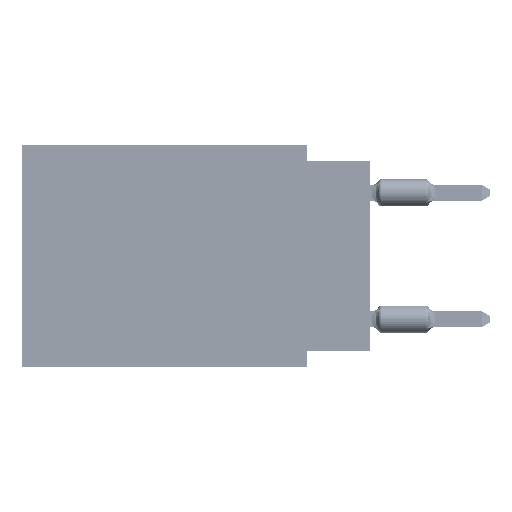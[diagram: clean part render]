
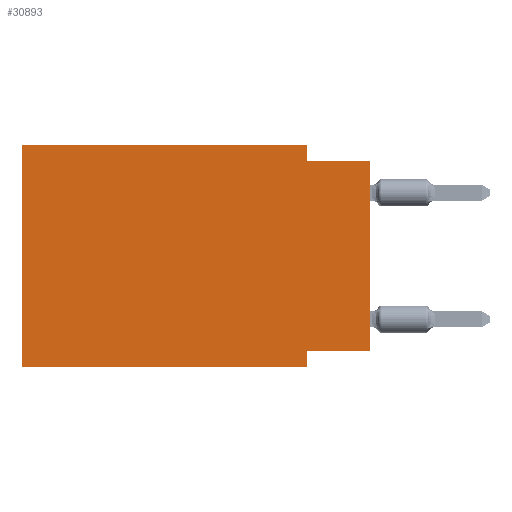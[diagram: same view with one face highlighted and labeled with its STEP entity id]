
A CAD part, left-side view. The second image highlights one B-rep face of the part: STEP entity #30893.
In plain terms, the highlighted planar face has unit normal (-1, 0, 0).
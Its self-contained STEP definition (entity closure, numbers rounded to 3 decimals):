
#2110 = CARTESIAN_POINT ( 'NONE',  ( 0., 2.54, -0.635 ) ) ;
#4095 = FACE_OUTER_BOUND ( 'NONE', #34956, .T. ) ;
#6099 = CARTESIAN_POINT ( 'NONE',  ( 0., 13.97, -8.89 ) ) ;
#6158 = CARTESIAN_POINT ( 'NONE',  ( 0., 2.54, 0. ) ) ;
#8607 = ORIENTED_EDGE ( 'NONE', *, *, #38742, .F. ) ;
#10817 = DIRECTION ( 'NONE',  ( 0., 0., -1. ) ) ;
#11396 = ORIENTED_EDGE ( 'NONE', *, *, #22420, .F. ) ;
#11753 = VECTOR ( 'NONE', #76436, 1000. ) ;
#12041 = LINE ( 'NONE', #6158, #82120 ) ;
#13299 = CARTESIAN_POINT ( 'NONE',  ( 0., 0., -0.635 ) ) ;
#13456 = DIRECTION ( 'NONE',  ( 0., -1., 0. ) ) ;
#13881 = LINE ( 'NONE', #44991, #46534 ) ;
#14516 = VERTEX_POINT ( 'NONE', #49540 ) ;
#15946 = VECTOR ( 'NONE', #69923, 1000. ) ;
#16169 = CARTESIAN_POINT ( 'NONE',  ( 0., 2.54, 0. ) ) ;
#17230 = LINE ( 'NONE', #75221, #55458 ) ;
#17736 = LINE ( 'NONE', #56386, #31628 ) ;
#20654 = CARTESIAN_POINT ( 'NONE',  ( 0., 2.54, -8.89 ) ) ;
#22420 = EDGE_CURVE ( 'NONE', #79474, #53829, #17230, .T. ) ;
#25163 = CARTESIAN_POINT ( 'NONE',  ( 0., 13.97, -8.89 ) ) ;
#25409 = VECTOR ( 'NONE', #31245, 1000. ) ;
#25682 = CARTESIAN_POINT ( 'NONE',  ( 0., 13.97, 0. ) ) ;
#26259 = EDGE_CURVE ( 'NONE', #60961, #70856, #13881, .T. ) ;
#28973 = EDGE_CURVE ( 'NONE', #14516, #79474, #46061, .T. ) ;
#29222 = ORIENTED_EDGE ( 'NONE', *, *, #26259, .F. ) ;
#29746 = PLANE ( 'NONE',  #76397 ) ;
#29866 = DIRECTION ( 'NONE',  ( 0., 0., -1. ) ) ;
#30893 = ADVANCED_FACE ( 'NONE', ( #4095 ), #29746, .F. ) ;
#30972 = DIRECTION ( 'NONE',  ( 0., 0., -1. ) ) ;
#31245 = DIRECTION ( 'NONE',  ( 0., -1., 0. ) ) ;
#31508 = ORIENTED_EDGE ( 'NONE', *, *, #77738, .T. ) ;
#31628 = VECTOR ( 'NONE', #68995, 1000. ) ;
#34956 = EDGE_LOOP ( 'NONE', ( #69501, #36332, #8607, #29222, #40381, #31508, #11396, #66861 ) ) ;
#36332 = ORIENTED_EDGE ( 'NONE', *, *, #47498, .F. ) ;
#37785 = LINE ( 'NONE', #25163, #11753 ) ;
#38623 = VERTEX_POINT ( 'NONE', #2110 ) ;
#38742 = EDGE_CURVE ( 'NONE', #70856, #38623, #12041, .T. ) ;
#40381 = ORIENTED_EDGE ( 'NONE', *, *, #75377, .F. ) ;
#42753 = DIRECTION ( 'NONE',  ( 1., 0., 0. ) ) ;
#43443 = CARTESIAN_POINT ( 'NONE',  ( 0., 0., -0.635 ) ) ;
#44651 = VERTEX_POINT ( 'NONE', #6099 ) ;
#44991 = CARTESIAN_POINT ( 'NONE',  ( 0., 13.97, 0. ) ) ;
#46061 = LINE ( 'NONE', #79217, #71001 ) ;
#46534 = VECTOR ( 'NONE', #13456, 1000. ) ;
#46897 = CARTESIAN_POINT ( 'NONE',  ( 0., 2.54, -8.255 ) ) ;
#47498 = EDGE_CURVE ( 'NONE', #38623, #49875, #76182, .T. ) ;
#49050 = CARTESIAN_POINT ( 'NONE',  ( 0., 13.97, 0. ) ) ;
#49540 = CARTESIAN_POINT ( 'NONE',  ( 0., 0., -8.255 ) ) ;
#49875 = VERTEX_POINT ( 'NONE', #13299 ) ;
#53829 = VERTEX_POINT ( 'NONE', #20654 ) ;
#55458 = VECTOR ( 'NONE', #29866, 1000. ) ;
#56386 = CARTESIAN_POINT ( 'NONE',  ( 0., 13.97, 0. ) ) ;
#56907 = CARTESIAN_POINT ( 'NONE',  ( 0., 0., 0. ) ) ;
#58223 = EDGE_CURVE ( 'NONE', #14516, #49875, #62775, .T. ) ;
#59493 = DIRECTION ( 'NONE',  ( 0., 1., 0. ) ) ;
#60961 = VERTEX_POINT ( 'NONE', #25682 ) ;
#62775 = LINE ( 'NONE', #56907, #15946 ) ;
#66861 = ORIENTED_EDGE ( 'NONE', *, *, #28973, .F. ) ;
#68995 = DIRECTION ( 'NONE',  ( 0., 0., 1. ) ) ;
#69501 = ORIENTED_EDGE ( 'NONE', *, *, #58223, .T. ) ;
#69923 = DIRECTION ( 'NONE',  ( 0., 0., 1. ) ) ;
#70856 = VERTEX_POINT ( 'NONE', #16169 ) ;
#71001 = VECTOR ( 'NONE', #59493, 1000. ) ;
#75221 = CARTESIAN_POINT ( 'NONE',  ( 0., 2.54, -8.89 ) ) ;
#75377 = EDGE_CURVE ( 'NONE', #44651, #60961, #17736, .T. ) ;
#76182 = LINE ( 'NONE', #43443, #25409 ) ;
#76397 = AXIS2_PLACEMENT_3D ( 'NONE', #49050, #42753, #10817 ) ;
#76436 = DIRECTION ( 'NONE',  ( 0., -1., 0. ) ) ;
#77738 = EDGE_CURVE ( 'NONE', #44651, #53829, #37785, .T. ) ;
#79217 = CARTESIAN_POINT ( 'NONE',  ( 0., 0., -8.255 ) ) ;
#79474 = VERTEX_POINT ( 'NONE', #46897 ) ;
#82120 = VECTOR ( 'NONE', #30972, 1000. ) ;
